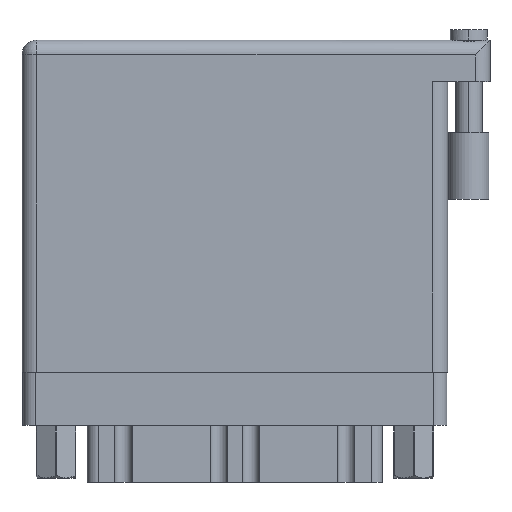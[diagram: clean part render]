
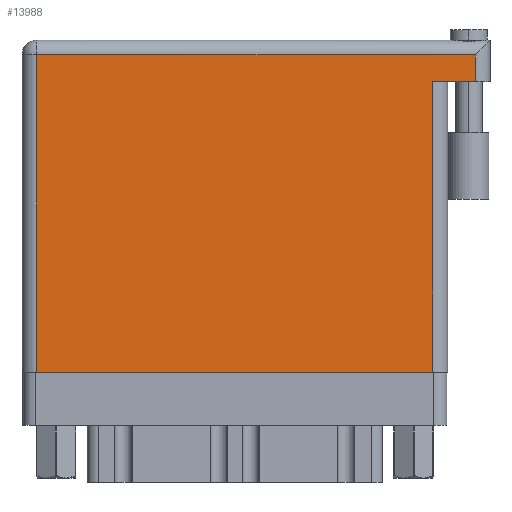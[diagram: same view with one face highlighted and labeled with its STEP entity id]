
A CAD part, front view. The second image highlights one B-rep face of the part: STEP entity #13988.
In plain terms, the highlighted face is planar.
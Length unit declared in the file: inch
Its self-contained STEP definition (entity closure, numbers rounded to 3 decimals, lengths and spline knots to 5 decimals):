
#843 = CARTESIAN_POINT ( 'NONE',  ( 1.938, 1.369, 0. ) ) ;
#1561 = VECTOR ( 'NONE', #34092, 39.37008 ) ;
#1574 = FACE_OUTER_BOUND ( 'NONE', #2453, .T. ) ;
#2340 = ORIENTED_EDGE ( 'NONE', *, *, #45448, .T. ) ;
#2453 = EDGE_LOOP ( 'NONE', ( #28788, #41804, #36897, #2340, #40936, #18955 ) ) ;
#2838 = DIRECTION ( 'NONE',  ( 0., 1., 0. ) ) ;
#3074 = LINE ( 'NONE', #843, #5797 ) ;
#3412 = VERTEX_POINT ( 'NONE', #15697 ) ;
#3965 = DIRECTION ( 'NONE',  ( 0., -1., 0. ) ) ;
#4294 = EDGE_CURVE ( 'NONE', #17835, #44668, #8030, .T. ) ;
#4587 = VECTOR ( 'NONE', #14240, 39.37008 ) ;
#5447 = AXIS2_PLACEMENT_3D ( 'NONE', #8747, #37836, #19955 ) ;
#5797 = VECTOR ( 'NONE', #2838, 39.37008 ) ;
#6856 = CARTESIAN_POINT ( 'NONE',  ( 0.07, 0., 0. ) ) ;
#8030 = LINE ( 'NONE', #40667, #23368 ) ;
#8747 = CARTESIAN_POINT ( 'NONE',  ( 0., 1.566, 0. ) ) ;
#11188 = CARTESIAN_POINT ( 'NONE',  ( 2.208, 1.369, 0. ) ) ;
#12292 = DIRECTION ( 'NONE',  ( -1., 0., 0. ) ) ;
#12762 = CARTESIAN_POINT ( 'NONE',  ( 1.938, 0., 0. ) ) ;
#13988 = ADVANCED_FACE ( 'NONE', ( #1574 ), #30650, .F. ) ;
#14240 = DIRECTION ( 'NONE',  ( 1., 0., 0. ) ) ;
#15697 = CARTESIAN_POINT ( 'NONE',  ( 2.138, 1.369, 0. ) ) ;
#16107 = LINE ( 'NONE', #44936, #32684 ) ;
#17645 = DIRECTION ( 'NONE',  ( -1., 0., 0. ) ) ;
#17835 = VERTEX_POINT ( 'NONE', #23209 ) ;
#18955 = ORIENTED_EDGE ( 'NONE', *, *, #4294, .T. ) ;
#19167 = CARTESIAN_POINT ( 'NONE',  ( 2.138, 1.496, 0. ) ) ;
#19955 = DIRECTION ( 'NONE',  ( -1., 0., 0. ) ) ;
#22662 = CARTESIAN_POINT ( 'NONE',  ( 2.138, 1.566, 0. ) ) ;
#22949 = CARTESIAN_POINT ( 'NONE',  ( 1.938, 1.369, 0. ) ) ;
#23209 = CARTESIAN_POINT ( 'NONE',  ( 0.07, 1.496, 0. ) ) ;
#23368 = VECTOR ( 'NONE', #3965, 39.37008 ) ;
#24952 = LINE ( 'NONE', #46886, #4587 ) ;
#25000 = LINE ( 'NONE', #11188, #31960 ) ;
#26552 = VERTEX_POINT ( 'NONE', #22949 ) ;
#27655 = EDGE_CURVE ( 'NONE', #31272, #26552, #3074, .T. ) ;
#28788 = ORIENTED_EDGE ( 'NONE', *, *, #44708, .T. ) ;
#30650 = PLANE ( 'NONE',  #5447 ) ;
#31127 = EDGE_CURVE ( 'NONE', #34022, #17835, #16107, .T. ) ;
#31272 = VERTEX_POINT ( 'NONE', #12762 ) ;
#31960 = VECTOR ( 'NONE', #17645, 39.37008 ) ;
#32684 = VECTOR ( 'NONE', #12292, 39.37008 ) ;
#34022 = VERTEX_POINT ( 'NONE', #19167 ) ;
#34092 = DIRECTION ( 'NONE',  ( 0., 1., 0. ) ) ;
#36897 = ORIENTED_EDGE ( 'NONE', *, *, #44008, .F. ) ;
#37836 = DIRECTION ( 'NONE',  ( 0., 0., -1. ) ) ;
#40667 = CARTESIAN_POINT ( 'NONE',  ( 0.07, 0., 0. ) ) ;
#40936 = ORIENTED_EDGE ( 'NONE', *, *, #31127, .T. ) ;
#40993 = LINE ( 'NONE', #22662, #1561 ) ;
#41804 = ORIENTED_EDGE ( 'NONE', *, *, #27655, .T. ) ;
#44008 = EDGE_CURVE ( 'NONE', #3412, #26552, #25000, .T. ) ;
#44668 = VERTEX_POINT ( 'NONE', #6856 ) ;
#44708 = EDGE_CURVE ( 'NONE', #44668, #31272, #24952, .T. ) ;
#44936 = CARTESIAN_POINT ( 'NONE',  ( 0., 1.496, 0. ) ) ;
#45448 = EDGE_CURVE ( 'NONE', #3412, #34022, #40993, .T. ) ;
#46886 = CARTESIAN_POINT ( 'NONE',  ( 0., 0., 0. ) ) ;
